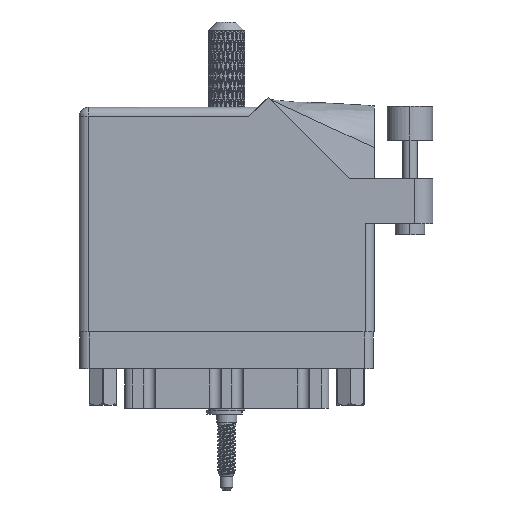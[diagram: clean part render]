
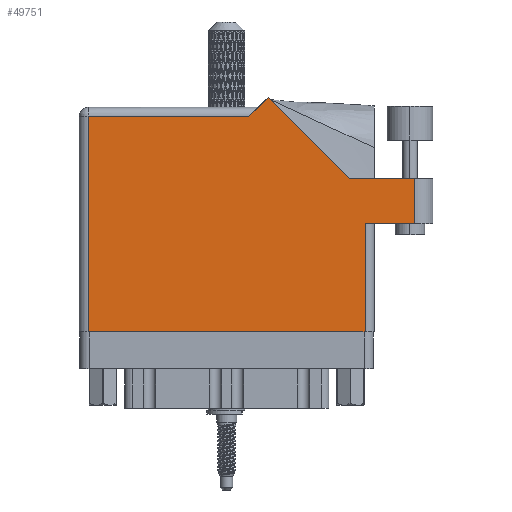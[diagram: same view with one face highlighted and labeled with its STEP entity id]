
A CAD part, front view. The second image highlights one B-rep face of the part: STEP entity #49751.
In plain terms, the highlighted face is planar.
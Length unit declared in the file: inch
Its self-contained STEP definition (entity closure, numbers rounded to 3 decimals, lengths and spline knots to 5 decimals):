
#1226 = LINE ( 'NONE', #36168, #5114 ) ;
#2317 = ORIENTED_EDGE ( 'NONE', *, *, #29009, .T. ) ;
#3137 = EDGE_CURVE ( 'NONE', #59000, #84448, #84020, .T. ) ;
#3713 = LINE ( 'NONE', #91965, #109676 ) ;
#5114 = VECTOR ( 'NONE', #71139, 39.37008 ) ;
#5218 = CARTESIAN_POINT ( 'NONE',  ( 0.062, 0., 0. ) ) ;
#7683 = EDGE_CURVE ( 'NONE', #95914, #38271, #19991, .T. ) ;
#10689 = CARTESIAN_POINT ( 'NONE',  ( 1.84442, 1.044, 0. ) ) ;
#11812 = VERTEX_POINT ( 'NONE', #5218 ) ;
#12017 = DIRECTION ( 'NONE',  ( -1., 0., 0. ) ) ;
#12411 = CARTESIAN_POINT ( 'NONE',  ( 2.285, 1.044, 0. ) ) ;
#13829 = ORIENTED_EDGE ( 'NONE', *, *, #7683, .T. ) ;
#14414 = ORIENTED_EDGE ( 'NONE', *, *, #46445, .T. ) ;
#14647 = DIRECTION ( 'NONE',  ( 0., 1., 0. ) ) ;
#16148 = DIRECTION ( 'NONE',  ( 1., 0., 0. ) ) ;
#17665 = EDGE_CURVE ( 'NONE', #20325, #11812, #61374, .T. ) ;
#19991 = LINE ( 'NONE', #28593, #109056 ) ;
#20325 = VERTEX_POINT ( 'NONE', #47531 ) ;
#20406 = ORIENTED_EDGE ( 'NONE', *, *, #3137, .T. ) ;
#21232 = VECTOR ( 'NONE', #109572, 39.37008 ) ;
#22007 = CARTESIAN_POINT ( 'NONE',  ( 1.948, 0.737, 0. ) ) ;
#23286 = EDGE_CURVE ( 'NONE', #103631, #20325, #82055, .T. ) ;
#23667 = ORIENTED_EDGE ( 'NONE', *, *, #56662, .T. ) ;
#25936 = CARTESIAN_POINT ( 'NONE',  ( 1.948, 0., 0. ) ) ;
#28593 = CARTESIAN_POINT ( 'NONE',  ( 1.948, 0.737, 0. ) ) ;
#28632 = LINE ( 'NONE', #63548, #42983 ) ;
#29009 = EDGE_CURVE ( 'NONE', #75689, #69155, #87403, .T. ) ;
#30668 = CARTESIAN_POINT ( 'NONE',  ( 0.062, 0., 0. ) ) ;
#31779 = DIRECTION ( 'NONE',  ( 0., -1., 0. ) ) ;
#36168 = CARTESIAN_POINT ( 'NONE',  ( 2.41, 1.044, 0. ) ) ;
#36680 = DIRECTION ( 'NONE',  ( 0., 0., -1. ) ) ;
#36683 = VECTOR ( 'NONE', #31779, 39.37008 ) ;
#38271 = VERTEX_POINT ( 'NONE', #22007 ) ;
#38485 = CARTESIAN_POINT ( 'NONE',  ( 0., 1.468, 0. ) ) ;
#38661 = DIRECTION ( 'NONE',  ( 1., 0., 0. ) ) ;
#38895 = CARTESIAN_POINT ( 'NONE',  ( 1.28771, 1.60071, 0. ) ) ;
#42824 = VECTOR ( 'NONE', #14647, 39.37008 ) ;
#42983 = VECTOR ( 'NONE', #98543, 39.37008 ) ;
#43632 = LINE ( 'NONE', #78018, #47600 ) ;
#43736 = AXIS2_PLACEMENT_3D ( 'NONE', #66808, #36680, #12017 ) ;
#46445 = EDGE_CURVE ( 'NONE', #84448, #75689, #1226, .T. ) ;
#47531 = CARTESIAN_POINT ( 'NONE',  ( 0.062, 1.468, 0. ) ) ;
#47600 = VECTOR ( 'NONE', #16148, 39.37008 ) ;
#47719 = ORIENTED_EDGE ( 'NONE', *, *, #23286, .T. ) ;
#49751 = ADVANCED_FACE ( 'NONE', ( #98582 ), #101815, .F. ) ;
#51718 = EDGE_CURVE ( 'NONE', #38271, #59000, #43632, .T. ) ;
#53255 = DIRECTION ( 'NONE',  ( 0., 1., 0. ) ) ;
#56662 = EDGE_CURVE ( 'NONE', #11812, #95914, #3713, .T. ) ;
#59000 = VERTEX_POINT ( 'NONE', #107140 ) ;
#59454 = ORIENTED_EDGE ( 'NONE', *, *, #69163, .T. ) ;
#60993 = DIRECTION ( 'NONE',  ( -0.707, 0.707, 0. ) ) ;
#61374 = LINE ( 'NONE', #30668, #36683 ) ;
#63548 = CARTESIAN_POINT ( 'NONE',  ( 1.217, 1.53, 0. ) ) ;
#63640 = CARTESIAN_POINT ( 'NONE',  ( 1.155, 1.468, 0. ) ) ;
#65637 = ORIENTED_EDGE ( 'NONE', *, *, #17665, .T. ) ;
#66808 = CARTESIAN_POINT ( 'NONE',  ( 0., 1.53, 0. ) ) ;
#67839 = VECTOR ( 'NONE', #60993, 39.37008 ) ;
#69155 = VERTEX_POINT ( 'NONE', #38895 ) ;
#69163 = EDGE_CURVE ( 'NONE', #69155, #103631, #28632, .T. ) ;
#71139 = DIRECTION ( 'NONE',  ( -1., 0., 0. ) ) ;
#75689 = VERTEX_POINT ( 'NONE', #10689 ) ;
#78018 = CARTESIAN_POINT ( 'NONE',  ( 2.01, 0.737, 0. ) ) ;
#82055 = LINE ( 'NONE', #38485, #21232 ) ;
#84020 = LINE ( 'NONE', #12411, #42824 ) ;
#84448 = VERTEX_POINT ( 'NONE', #85942 ) ;
#85942 = CARTESIAN_POINT ( 'NONE',  ( 2.285, 1.044, 0. ) ) ;
#87403 = LINE ( 'NONE', #94862, #67839 ) ;
#91965 = CARTESIAN_POINT ( 'NONE',  ( 0., 0., 0. ) ) ;
#92502 = ORIENTED_EDGE ( 'NONE', *, *, #51718, .T. ) ;
#94862 = CARTESIAN_POINT ( 'NONE',  ( 1.84442, 1.044, 0. ) ) ;
#95914 = VERTEX_POINT ( 'NONE', #25936 ) ;
#98543 = DIRECTION ( 'NONE',  ( -0.707, -0.707, 0. ) ) ;
#98582 = FACE_OUTER_BOUND ( 'NONE', #103026, .T. ) ;
#101815 = PLANE ( 'NONE',  #43736 ) ;
#103026 = EDGE_LOOP ( 'NONE', ( #92502, #20406, #14414, #2317, #59454, #47719, #65637, #23667, #13829 ) ) ;
#103631 = VERTEX_POINT ( 'NONE', #63640 ) ;
#107140 = CARTESIAN_POINT ( 'NONE',  ( 2.285, 0.737, 0. ) ) ;
#109056 = VECTOR ( 'NONE', #53255, 39.37008 ) ;
#109572 = DIRECTION ( 'NONE',  ( -1., 0., 0. ) ) ;
#109676 = VECTOR ( 'NONE', #38661, 39.37008 ) ;
